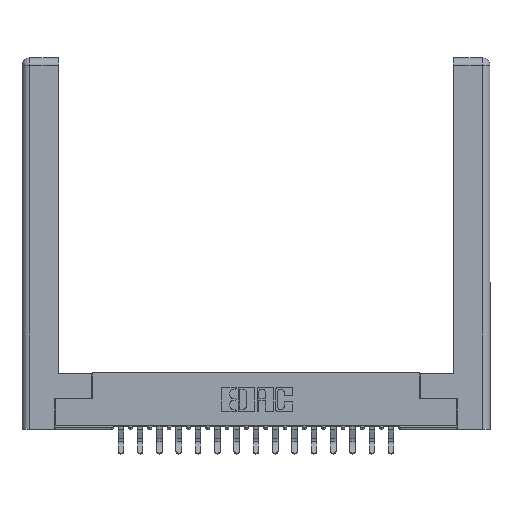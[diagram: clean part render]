
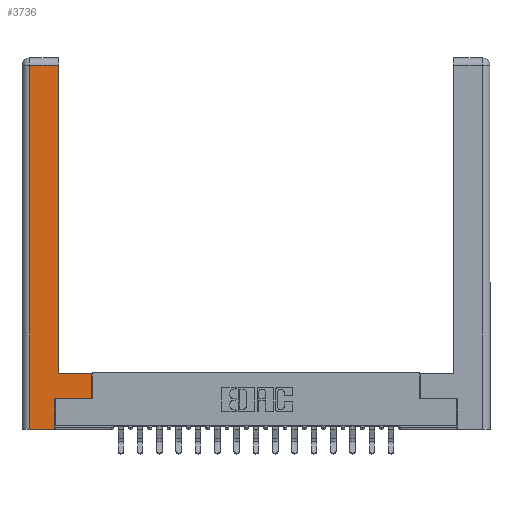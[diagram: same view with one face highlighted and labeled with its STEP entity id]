
A CAD part, top view. The second image highlights one B-rep face of the part: STEP entity #3736.
In plain terms, the highlighted planar face has unit normal (0, 0, 1).
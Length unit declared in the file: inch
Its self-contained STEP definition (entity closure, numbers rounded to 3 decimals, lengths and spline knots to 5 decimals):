
#177 = EDGE_LOOP ( 'NONE', ( #9502, #1821, #13983, #18258, #4123, #12535, #21040, #10687 ) ) ;
#534 = CARTESIAN_POINT ( 'NONE',  ( 0.0615, 0., 0. ) ) ;
#548 = LINE ( 'NONE', #14548, #18401 ) ;
#913 = VECTOR ( 'NONE', #9063, 39.37008 ) ;
#917 = CARTESIAN_POINT ( 'NONE',  ( 0.565, 0.45, 0. ) ) ;
#1821 = ORIENTED_EDGE ( 'NONE', *, *, #19018, .T. ) ;
#2052 = CARTESIAN_POINT ( 'NONE',  ( 0.565, 0.245, 0. ) ) ;
#2871 = LINE ( 'NONE', #15367, #19658 ) ;
#3085 = LINE ( 'NONE', #2052, #913 ) ;
#3520 = FACE_OUTER_BOUND ( 'NONE', #177, .T. ) ;
#3736 = ADVANCED_FACE ( 'NONE', ( #3520 ), #14250, .F. ) ;
#4123 = ORIENTED_EDGE ( 'NONE', *, *, #15854, .T. ) ;
#4344 = CARTESIAN_POINT ( 'NONE',  ( 0.0615, 0., 0. ) ) ;
#5964 = LINE ( 'NONE', #16898, #16797 ) ;
#6037 = CARTESIAN_POINT ( 'NONE',  ( 0.0615, 2.94, 0. ) ) ;
#6088 = DIRECTION ( 'NONE',  ( 0., -1., 0. ) ) ;
#6414 = CARTESIAN_POINT ( 'NONE',  ( 0.295, 0.45, 0. ) ) ;
#6487 = VERTEX_POINT ( 'NONE', #534 ) ;
#6531 = DIRECTION ( 'NONE',  ( 0., 1., 0. ) ) ;
#7189 = CARTESIAN_POINT ( 'NONE',  ( 0.265, 0., 0. ) ) ;
#7880 = VECTOR ( 'NONE', #6088, 39.37008 ) ;
#8506 = LINE ( 'NONE', #917, #20458 ) ;
#9063 = DIRECTION ( 'NONE',  ( 1., 0., 0. ) ) ;
#9161 = DIRECTION ( 'NONE',  ( 0., 0., -1. ) ) ;
#9502 = ORIENTED_EDGE ( 'NONE', *, *, #11676, .T. ) ;
#9783 = DIRECTION ( 'NONE',  ( -1., 0., 0. ) ) ;
#9810 = DIRECTION ( 'NONE',  ( 0., 1., 0. ) ) ;
#9855 = VERTEX_POINT ( 'NONE', #13645 ) ;
#9911 = LINE ( 'NONE', #7189, #12336 ) ;
#10323 = VERTEX_POINT ( 'NONE', #15176 ) ;
#10645 = DIRECTION ( 'NONE',  ( 1., 0., 0. ) ) ;
#10687 = ORIENTED_EDGE ( 'NONE', *, *, #16744, .T. ) ;
#11139 = EDGE_CURVE ( 'NONE', #6487, #21178, #9911, .T. ) ;
#11676 = EDGE_CURVE ( 'NONE', #9855, #14947, #2871, .T. ) ;
#12336 = VECTOR ( 'NONE', #10645, 39.37008 ) ;
#12356 = CARTESIAN_POINT ( 'NONE',  ( 0.565, 0.45, 0. ) ) ;
#12450 = CARTESIAN_POINT ( 'NONE',  ( 0.295, 2.94, 0. ) ) ;
#12535 = ORIENTED_EDGE ( 'NONE', *, *, #13684, .T. ) ;
#13150 = VERTEX_POINT ( 'NONE', #12356 ) ;
#13203 = VERTEX_POINT ( 'NONE', #15778 ) ;
#13645 = CARTESIAN_POINT ( 'NONE',  ( 0.295, 0.45, 0. ) ) ;
#13684 = EDGE_CURVE ( 'NONE', #13203, #10323, #3085, .T. ) ;
#13725 = CARTESIAN_POINT ( 'NONE',  ( 0.265, 0., 0. ) ) ;
#13983 = ORIENTED_EDGE ( 'NONE', *, *, #18086, .T. ) ;
#14250 = PLANE ( 'NONE',  #15919 ) ;
#14548 = CARTESIAN_POINT ( 'NONE',  ( 0.0615, 2.94, 0. ) ) ;
#14947 = VERTEX_POINT ( 'NONE', #12450 ) ;
#15066 = VERTEX_POINT ( 'NONE', #6037 ) ;
#15176 = CARTESIAN_POINT ( 'NONE',  ( 0.565, 0.245, 0. ) ) ;
#15367 = CARTESIAN_POINT ( 'NONE',  ( 0.295, 3., 0. ) ) ;
#15778 = CARTESIAN_POINT ( 'NONE',  ( 0.265, 0.245, 0. ) ) ;
#15827 = DIRECTION ( 'NONE',  ( -1., 0., 0. ) ) ;
#15854 = EDGE_CURVE ( 'NONE', #21178, #13203, #5964, .T. ) ;
#15919 = AXIS2_PLACEMENT_3D ( 'NONE', #17716, #9161, #15827 ) ;
#16522 = EDGE_CURVE ( 'NONE', #10323, #13150, #8506, .T. ) ;
#16744 = EDGE_CURVE ( 'NONE', #13150, #9855, #20969, .T. ) ;
#16797 = VECTOR ( 'NONE', #6531, 39.37008 ) ;
#16898 = CARTESIAN_POINT ( 'NONE',  ( 0.265, 0.245, 0. ) ) ;
#17716 = CARTESIAN_POINT ( 'NONE',  ( 0., 0., 0. ) ) ;
#18086 = EDGE_CURVE ( 'NONE', #15066, #6487, #22268, .T. ) ;
#18154 = DIRECTION ( 'NONE',  ( -1., 0., 0. ) ) ;
#18258 = ORIENTED_EDGE ( 'NONE', *, *, #11139, .T. ) ;
#18401 = VECTOR ( 'NONE', #18154, 39.37008 ) ;
#18686 = DIRECTION ( 'NONE',  ( 0., 1., 0. ) ) ;
#19018 = EDGE_CURVE ( 'NONE', #14947, #15066, #548, .T. ) ;
#19658 = VECTOR ( 'NONE', #18686, 39.37008 ) ;
#20458 = VECTOR ( 'NONE', #9810, 39.37008 ) ;
#20696 = VECTOR ( 'NONE', #9783, 39.37008 ) ;
#20969 = LINE ( 'NONE', #6414, #20696 ) ;
#21040 = ORIENTED_EDGE ( 'NONE', *, *, #16522, .T. ) ;
#21178 = VERTEX_POINT ( 'NONE', #13725 ) ;
#22268 = LINE ( 'NONE', #4344, #7880 ) ;
